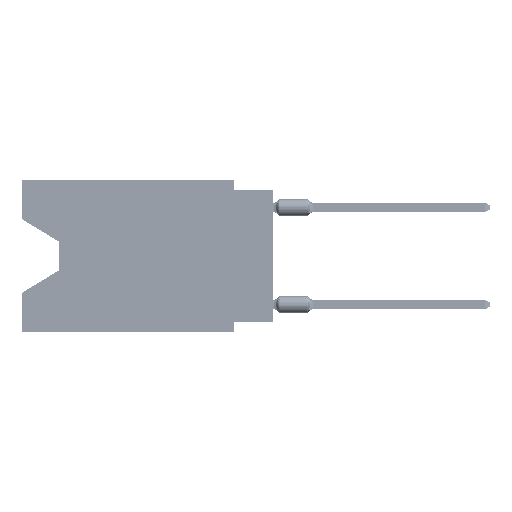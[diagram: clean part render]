
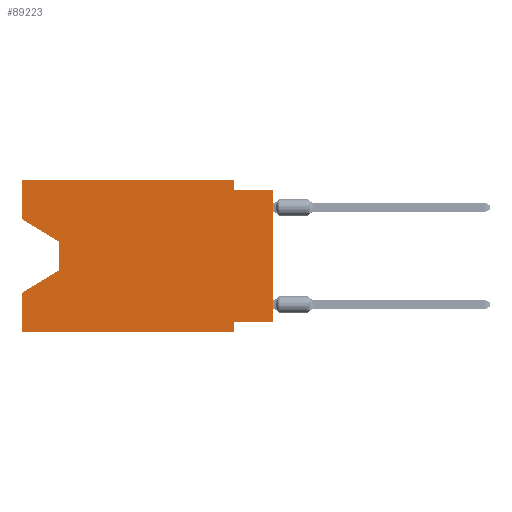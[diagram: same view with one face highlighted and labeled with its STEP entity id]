
A CAD part, left-side view. The second image highlights one B-rep face of the part: STEP entity #89223.
In plain terms, the highlighted planar face has unit normal (-1, 0, 0).
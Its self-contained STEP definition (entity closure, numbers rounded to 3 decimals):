
#755 = DIRECTION ( 'NONE',  ( 0., -0.855, -0.519 ) ) ;
#1051 = DIRECTION ( 'NONE',  ( 0., 0., 1. ) ) ;
#1782 = LINE ( 'NONE', #83815, #51003 ) ;
#2376 = EDGE_CURVE ( 'NONE', #44219, #7906, #1782, .T. ) ;
#2579 = DIRECTION ( 'NONE',  ( 0., 0., 1. ) ) ;
#2952 = VERTEX_POINT ( 'NONE', #59939 ) ;
#4829 = VERTEX_POINT ( 'NONE', #87821 ) ;
#6945 = FACE_OUTER_BOUND ( 'NONE', #56181, .T. ) ;
#7593 = LINE ( 'NONE', #35825, #79917 ) ;
#7890 = LINE ( 'NONE', #63484, #57587 ) ;
#7906 = VERTEX_POINT ( 'NONE', #70709 ) ;
#8294 = DIRECTION ( 'NONE',  ( 0., 0., -1. ) ) ;
#8527 = CARTESIAN_POINT ( 'NONE',  ( 0., 16.383, 0. ) ) ;
#8528 = VERTEX_POINT ( 'NONE', #39087 ) ;
#9043 = CARTESIAN_POINT ( 'NONE',  ( 0., 16.383, -7.36 ) ) ;
#9081 = LINE ( 'NONE', #65571, #50497 ) ;
#10238 = VECTOR ( 'NONE', #88678, 1000. ) ;
#11040 = VECTOR ( 'NONE', #13930, 1000. ) ;
#11304 = EDGE_CURVE ( 'NONE', #52472, #79863, #49945, .T. ) ;
#13930 = DIRECTION ( 'NONE',  ( 0., -1., 0. ) ) ;
#14839 = LINE ( 'NONE', #41736, #11040 ) ;
#15716 = DIRECTION ( 'NONE',  ( 0., 1., 0. ) ) ;
#16021 = LINE ( 'NONE', #53363, #21747 ) ;
#16540 = VERTEX_POINT ( 'NONE', #83015 ) ;
#18828 = ORIENTED_EDGE ( 'NONE', *, *, #56097, .T. ) ;
#20765 = LINE ( 'NONE', #54073, #10238 ) ;
#21747 = VECTOR ( 'NONE', #87965, 1000. ) ;
#22942 = EDGE_CURVE ( 'NONE', #4829, #16540, #60869, .T. ) ;
#23210 = ORIENTED_EDGE ( 'NONE', *, *, #83625, .F. ) ;
#25403 = ORIENTED_EDGE ( 'NONE', *, *, #78414, .F. ) ;
#28305 = VERTEX_POINT ( 'NONE', #9043 ) ;
#31812 = AXIS2_PLACEMENT_3D ( 'NONE', #77559, #70731, #8294 ) ;
#32551 = VERTEX_POINT ( 'NONE', #70142 ) ;
#33236 = ORIENTED_EDGE ( 'NONE', *, *, #51520, .T. ) ;
#35825 = CARTESIAN_POINT ( 'NONE',  ( 0., 16.383, -2.546 ) ) ;
#38647 = VECTOR ( 'NONE', #2579, 1000. ) ;
#38699 = ORIENTED_EDGE ( 'NONE', *, *, #65617, .F. ) ;
#39087 = CARTESIAN_POINT ( 'NONE',  ( 0., 16.383, -2.546 ) ) ;
#41504 = VECTOR ( 'NONE', #15716, 1000. ) ;
#41736 = CARTESIAN_POINT ( 'NONE',  ( 0., 0., -0.635 ) ) ;
#42132 = LINE ( 'NONE', #43031, #43404 ) ;
#42522 = LINE ( 'NONE', #63037, #51758 ) ;
#42873 = ORIENTED_EDGE ( 'NONE', *, *, #88754, .T. ) ;
#43031 = CARTESIAN_POINT ( 'NONE',  ( 0., 0., 0. ) ) ;
#43404 = VECTOR ( 'NONE', #64438, 1000. ) ;
#44219 = VERTEX_POINT ( 'NONE', #85647 ) ;
#44851 = EDGE_CURVE ( 'NONE', #81890, #2952, #14839, .T. ) ;
#46198 = VERTEX_POINT ( 'NONE', #84107 ) ;
#46756 = CARTESIAN_POINT ( 'NONE',  ( 0., 16.383, -9.906 ) ) ;
#47611 = ORIENTED_EDGE ( 'NONE', *, *, #44851, .F. ) ;
#49781 = PLANE ( 'NONE',  #31812 ) ;
#49945 = LINE ( 'NONE', #84539, #41504 ) ;
#50497 = VECTOR ( 'NONE', #57390, 1000. ) ;
#51003 = VECTOR ( 'NONE', #57803, 1000. ) ;
#51520 = EDGE_CURVE ( 'NONE', #7906, #28305, #20765, .T. ) ;
#51603 = VECTOR ( 'NONE', #67728, 1000. ) ;
#51758 = VECTOR ( 'NONE', #83540, 1000. ) ;
#52472 = VERTEX_POINT ( 'NONE', #82081 ) ;
#53363 = CARTESIAN_POINT ( 'NONE',  ( 0., 2.54, -9.906 ) ) ;
#54073 = CARTESIAN_POINT ( 'NONE',  ( 0., 13.97, -5.893 ) ) ;
#56097 = EDGE_CURVE ( 'NONE', #8528, #44219, #7593, .T. ) ;
#56181 = EDGE_LOOP ( 'NONE', ( #18828, #71287, #33236, #23210, #58079, #87893, #63347, #42873, #47611, #25403, #38699, #78866 ) ) ;
#57390 = DIRECTION ( 'NONE',  ( 0., 0., -1. ) ) ;
#57587 = VECTOR ( 'NONE', #1051, 1000. ) ;
#57803 = DIRECTION ( 'NONE',  ( 0., 0., -1. ) ) ;
#58079 = ORIENTED_EDGE ( 'NONE', *, *, #22942, .T. ) ;
#59939 = CARTESIAN_POINT ( 'NONE',  ( 0., 0., -0.635 ) ) ;
#60869 = LINE ( 'NONE', #46756, #51603 ) ;
#61225 = CARTESIAN_POINT ( 'NONE',  ( 0., 2.54, -9.271 ) ) ;
#63037 = CARTESIAN_POINT ( 'NONE',  ( 0., 16.383, 0. ) ) ;
#63347 = ORIENTED_EDGE ( 'NONE', *, *, #11304, .F. ) ;
#63484 = CARTESIAN_POINT ( 'NONE',  ( 0., 16.383, 0. ) ) ;
#64438 = DIRECTION ( 'NONE',  ( 0., 0., 1. ) ) ;
#65571 = CARTESIAN_POINT ( 'NONE',  ( 0., 2.54, 0. ) ) ;
#65617 = EDGE_CURVE ( 'NONE', #46198, #32551, #42522, .T. ) ;
#67728 = DIRECTION ( 'NONE',  ( 0., -1., 0. ) ) ;
#67778 = CARTESIAN_POINT ( 'NONE',  ( 0., 2.54, -0.635 ) ) ;
#70142 = CARTESIAN_POINT ( 'NONE',  ( 0., 2.54, 0. ) ) ;
#70709 = CARTESIAN_POINT ( 'NONE',  ( 0., 13.97, -5.893 ) ) ;
#70731 = DIRECTION ( 'NONE',  ( 1., 0., 0. ) ) ;
#71287 = ORIENTED_EDGE ( 'NONE', *, *, #2376, .T. ) ;
#74875 = EDGE_CURVE ( 'NONE', #8528, #46198, #85954, .T. ) ;
#77559 = CARTESIAN_POINT ( 'NONE',  ( 0., 16.383, 0. ) ) ;
#78414 = EDGE_CURVE ( 'NONE', #32551, #81890, #9081, .T. ) ;
#78866 = ORIENTED_EDGE ( 'NONE', *, *, #74875, .F. ) ;
#79863 = VERTEX_POINT ( 'NONE', #61225 ) ;
#79917 = VECTOR ( 'NONE', #755, 1000. ) ;
#81890 = VERTEX_POINT ( 'NONE', #67778 ) ;
#82081 = CARTESIAN_POINT ( 'NONE',  ( 0., 0., -9.271 ) ) ;
#83015 = CARTESIAN_POINT ( 'NONE',  ( 0., 2.54, -9.906 ) ) ;
#83540 = DIRECTION ( 'NONE',  ( 0., -1., 0. ) ) ;
#83625 = EDGE_CURVE ( 'NONE', #4829, #28305, #7890, .T. ) ;
#83815 = CARTESIAN_POINT ( 'NONE',  ( 0., 13.97, -4.013 ) ) ;
#84107 = CARTESIAN_POINT ( 'NONE',  ( 0., 16.383, 0. ) ) ;
#84539 = CARTESIAN_POINT ( 'NONE',  ( 0., 0., -9.271 ) ) ;
#85647 = CARTESIAN_POINT ( 'NONE',  ( 0., 13.97, -4.013 ) ) ;
#85954 = LINE ( 'NONE', #8527, #38647 ) ;
#87821 = CARTESIAN_POINT ( 'NONE',  ( 0., 16.383, -9.906 ) ) ;
#87893 = ORIENTED_EDGE ( 'NONE', *, *, #89360, .F. ) ;
#87965 = DIRECTION ( 'NONE',  ( 0., 0., -1. ) ) ;
#88678 = DIRECTION ( 'NONE',  ( 0., 0.855, -0.519 ) ) ;
#88754 = EDGE_CURVE ( 'NONE', #52472, #2952, #42132, .T. ) ;
#89223 = ADVANCED_FACE ( 'NONE', ( #6945 ), #49781, .F. ) ;
#89360 = EDGE_CURVE ( 'NONE', #79863, #16540, #16021, .T. ) ;
